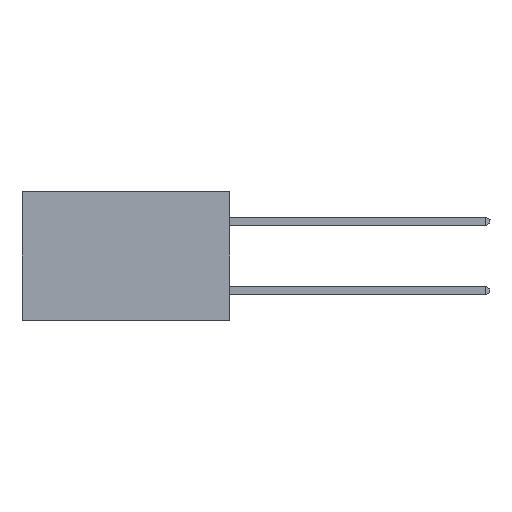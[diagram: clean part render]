
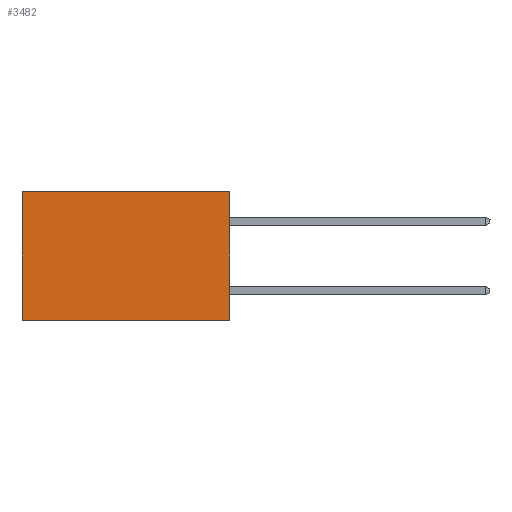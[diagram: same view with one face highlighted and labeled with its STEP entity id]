
A CAD part, left-side view. The second image highlights one B-rep face of the part: STEP entity #3482.
In plain terms, the highlighted planar face has unit normal (-1, 0, 0).
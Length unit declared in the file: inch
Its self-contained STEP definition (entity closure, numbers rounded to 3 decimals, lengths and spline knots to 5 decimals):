
#154 = VECTOR ( 'NONE', #4707, 39.37008 ) ;
#157 = EDGE_CURVE ( 'NONE', #8229, #14383, #4923, .T. ) ;
#426 = EDGE_CURVE ( 'NONE', #5601, #14383, #20399, .T. ) ;
#791 = EDGE_CURVE ( 'NONE', #2940, #8229, #17105, .T. ) ;
#2550 = DIRECTION ( 'NONE',  ( 0., 0., -1. ) ) ;
#2825 = AXIS2_PLACEMENT_3D ( 'NONE', #17955, #8583, #2550 ) ;
#2940 = VERTEX_POINT ( 'NONE', #3019 ) ;
#3019 = CARTESIAN_POINT ( 'NONE',  ( 0.298, 0., 0. ) ) ;
#3482 = ADVANCED_FACE ( 'NONE', ( #5770 ), #9861, .F. ) ;
#4707 = DIRECTION ( 'NONE',  ( 0., 1., 0. ) ) ;
#4923 = LINE ( 'NONE', #16372, #14651 ) ;
#5601 = VERTEX_POINT ( 'NONE', #6993 ) ;
#5770 = FACE_OUTER_BOUND ( 'NONE', #9517, .T. ) ;
#6993 = CARTESIAN_POINT ( 'NONE',  ( 0.298, 0., -0.37 ) ) ;
#7348 = DIRECTION ( 'NONE',  ( 0., 1., 0. ) ) ;
#8229 = VERTEX_POINT ( 'NONE', #15935 ) ;
#8583 = DIRECTION ( 'NONE',  ( 1., 0., 0. ) ) ;
#9077 = EDGE_CURVE ( 'NONE', #2940, #5601, #10458, .T. ) ;
#9517 = EDGE_LOOP ( 'NONE', ( #13289, #14775, #13405, #13477 ) ) ;
#9861 = PLANE ( 'NONE',  #2825 ) ;
#10458 = LINE ( 'NONE', #13690, #14720 ) ;
#10598 = DIRECTION ( 'NONE',  ( 0., 0., -1. ) ) ;
#13289 = ORIENTED_EDGE ( 'NONE', *, *, #157, .T. ) ;
#13405 = ORIENTED_EDGE ( 'NONE', *, *, #9077, .F. ) ;
#13477 = ORIENTED_EDGE ( 'NONE', *, *, #791, .T. ) ;
#13690 = CARTESIAN_POINT ( 'NONE',  ( 0.298, 0., 0. ) ) ;
#14130 = VECTOR ( 'NONE', #7348, 39.37008 ) ;
#14383 = VERTEX_POINT ( 'NONE', #16056 ) ;
#14651 = VECTOR ( 'NONE', #18035, 39.37008 ) ;
#14720 = VECTOR ( 'NONE', #10598, 39.37008 ) ;
#14775 = ORIENTED_EDGE ( 'NONE', *, *, #426, .F. ) ;
#15935 = CARTESIAN_POINT ( 'NONE',  ( 0.298, 0.6, 0. ) ) ;
#16056 = CARTESIAN_POINT ( 'NONE',  ( 0.298, 0.6, -0.37 ) ) ;
#16372 = CARTESIAN_POINT ( 'NONE',  ( 0.298, 0.6, 0. ) ) ;
#17105 = LINE ( 'NONE', #20360, #14130 ) ;
#17955 = CARTESIAN_POINT ( 'NONE',  ( 0.298, 0., 0. ) ) ;
#18035 = DIRECTION ( 'NONE',  ( 0., 0., -1. ) ) ;
#19019 = CARTESIAN_POINT ( 'NONE',  ( 0.298, 0., -0.37 ) ) ;
#20360 = CARTESIAN_POINT ( 'NONE',  ( 0.298, 0., 0. ) ) ;
#20399 = LINE ( 'NONE', #19019, #154 ) ;
